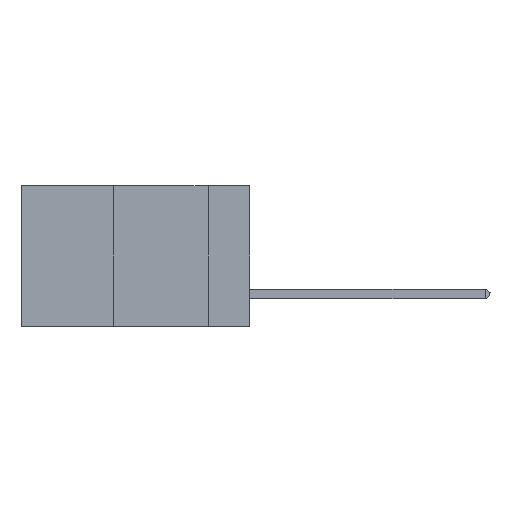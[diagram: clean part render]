
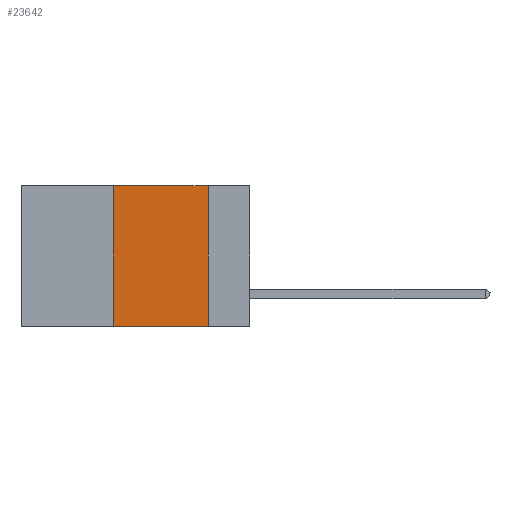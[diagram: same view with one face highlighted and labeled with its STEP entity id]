
A CAD part, left-side view. The second image highlights one B-rep face of the part: STEP entity #23642.
In plain terms, the highlighted planar face has unit normal (-1, 0, 0).
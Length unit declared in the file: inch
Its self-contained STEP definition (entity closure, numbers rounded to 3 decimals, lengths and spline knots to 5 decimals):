
#1666 = DIRECTION ( 'NONE',  ( 0., 0., 1. ) ) ;
#4448 = CARTESIAN_POINT ( 'NONE',  ( 0., 0.36, 0. ) ) ;
#6204 = VECTOR ( 'NONE', #18133, 39.37008 ) ;
#6398 = VECTOR ( 'NONE', #30476, 39.37008 ) ;
#8173 = EDGE_CURVE ( 'NONE', #35892, #26533, #24214, .T. ) ;
#8286 = CARTESIAN_POINT ( 'NONE',  ( 0., 0.6, 0. ) ) ;
#8932 = EDGE_CURVE ( 'NONE', #33358, #26533, #12707, .T. ) ;
#9283 = CARTESIAN_POINT ( 'NONE',  ( 0., 0.6, -0.37 ) ) ;
#11338 = LINE ( 'NONE', #4448, #30236 ) ;
#12707 = LINE ( 'NONE', #38208, #22189 ) ;
#17385 = PLANE ( 'NONE',  #25014 ) ;
#17520 = DIRECTION ( 'NONE',  ( 1., 0., 0. ) ) ;
#18133 = DIRECTION ( 'NONE',  ( 0., -1., 0. ) ) ;
#18507 = CARTESIAN_POINT ( 'NONE',  ( 0., 0.36, -0.37 ) ) ;
#20160 = ORIENTED_EDGE ( 'NONE', *, *, #37684, .F. ) ;
#20854 = CARTESIAN_POINT ( 'NONE',  ( 0., 0.11, -0.37 ) ) ;
#20945 = EDGE_LOOP ( 'NONE', ( #27585, #20160, #22922, #36367 ) ) ;
#22189 = VECTOR ( 'NONE', #25756, 39.37008 ) ;
#22922 = ORIENTED_EDGE ( 'NONE', *, *, #28783, .F. ) ;
#23642 = ADVANCED_FACE ( 'NONE', ( #34922 ), #17385, .F. ) ;
#24214 = LINE ( 'NONE', #9283, #6204 ) ;
#25014 = AXIS2_PLACEMENT_3D ( 'NONE', #8286, #17520, #29134 ) ;
#25756 = DIRECTION ( 'NONE',  ( 0., 0., -1. ) ) ;
#26533 = VERTEX_POINT ( 'NONE', #20854 ) ;
#27585 = ORIENTED_EDGE ( 'NONE', *, *, #8932, .F. ) ;
#27691 = VERTEX_POINT ( 'NONE', #33011 ) ;
#28783 = EDGE_CURVE ( 'NONE', #35892, #27691, #11338, .T. ) ;
#29134 = DIRECTION ( 'NONE',  ( 0., 0., -1. ) ) ;
#30236 = VECTOR ( 'NONE', #1666, 39.37008 ) ;
#30476 = DIRECTION ( 'NONE',  ( 0., -1., 0. ) ) ;
#30713 = CARTESIAN_POINT ( 'NONE',  ( 0., 0.11, 0. ) ) ;
#33011 = CARTESIAN_POINT ( 'NONE',  ( 0., 0.36, 0. ) ) ;
#33358 = VERTEX_POINT ( 'NONE', #30713 ) ;
#34277 = LINE ( 'NONE', #36988, #6398 ) ;
#34922 = FACE_OUTER_BOUND ( 'NONE', #20945, .T. ) ;
#35892 = VERTEX_POINT ( 'NONE', #18507 ) ;
#36367 = ORIENTED_EDGE ( 'NONE', *, *, #8173, .T. ) ;
#36988 = CARTESIAN_POINT ( 'NONE',  ( 0., 0.6, 0. ) ) ;
#37684 = EDGE_CURVE ( 'NONE', #27691, #33358, #34277, .T. ) ;
#38208 = CARTESIAN_POINT ( 'NONE',  ( 0., 0.11, 0. ) ) ;
